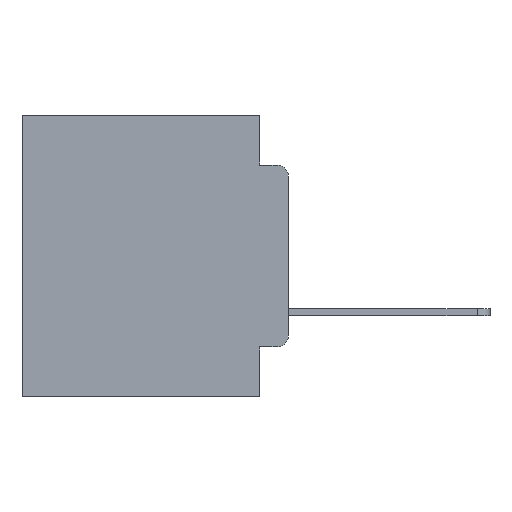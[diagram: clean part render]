
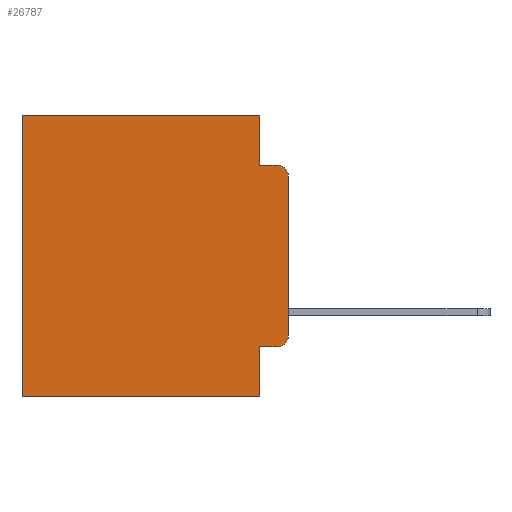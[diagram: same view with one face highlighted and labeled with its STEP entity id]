
A CAD part, left-side view. The second image highlights one B-rep face of the part: STEP entity #26787.
In plain terms, the highlighted planar face has unit normal (-1, 0, 0).
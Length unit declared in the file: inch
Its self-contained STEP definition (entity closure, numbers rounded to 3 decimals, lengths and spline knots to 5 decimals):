
#44 = CARTESIAN_POINT ( 'NONE',  ( 0.298, 0., -0.5 ) ) ;
#45 = EDGE_CURVE ( 'NONE', #5081, #11449, #20028, .T. ) ;
#139 = DIRECTION ( 'NONE',  ( 0., 1., 0. ) ) ;
#180 = VERTEX_POINT ( 'NONE', #13014 ) ;
#306 = ORIENTED_EDGE ( 'NONE', *, *, #12831, .F. ) ;
#857 = EDGE_CURVE ( 'NONE', #6445, #17383, #17025, .T. ) ;
#1104 = VECTOR ( 'NONE', #11165, 39.37008 ) ;
#1375 = VERTEX_POINT ( 'NONE', #20201 ) ;
#2165 = VECTOR ( 'NONE', #139, 39.37008 ) ;
#2789 = CARTESIAN_POINT ( 'NONE',  ( 0.298, 0., -0.3915 ) ) ;
#2856 = LINE ( 'NONE', #44, #2165 ) ;
#3295 = EDGE_CURVE ( 'NONE', #11449, #10520, #14204, .T. ) ;
#4187 = CIRCLE ( 'NONE', #17634, 0.02 ) ;
#4429 = AXIS2_PLACEMENT_3D ( 'NONE', #17873, #19975, #7284 ) ;
#5081 = VERTEX_POINT ( 'NONE', #22163 ) ;
#5127 = FACE_OUTER_BOUND ( 'NONE', #22429, .T. ) ;
#5281 = CARTESIAN_POINT ( 'NONE',  ( 0.298, 0.02, -0.4115 ) ) ;
#5890 = DIRECTION ( 'NONE',  ( 0., -1., 0. ) ) ;
#5969 = CARTESIAN_POINT ( 'NONE',  ( 0.298, 0., 0. ) ) ;
#6206 = ORIENTED_EDGE ( 'NONE', *, *, #22382, .F. ) ;
#6445 = VERTEX_POINT ( 'NONE', #11543 ) ;
#6539 = DIRECTION ( 'NONE',  ( 0., 1., 0. ) ) ;
#6581 = ORIENTED_EDGE ( 'NONE', *, *, #3295, .T. ) ;
#6962 = VECTOR ( 'NONE', #25093, 39.37008 ) ;
#7270 = DIRECTION ( 'NONE',  ( 0., 0., -1. ) ) ;
#7284 = DIRECTION ( 'NONE',  ( 0., 0., -1. ) ) ;
#7630 = LINE ( 'NONE', #10221, #6962 ) ;
#8241 = EDGE_CURVE ( 'NONE', #6445, #21262, #14792, .T. ) ;
#8368 = VERTEX_POINT ( 'NONE', #2789 ) ;
#8591 = EDGE_CURVE ( 'NONE', #180, #22905, #16775, .T. ) ;
#8826 = CARTESIAN_POINT ( 'NONE',  ( 0.298, 0.02, -0.0885 ) ) ;
#8924 = DIRECTION ( 'NONE',  ( -1., 0., 0. ) ) ;
#9073 = CARTESIAN_POINT ( 'NONE',  ( 0.298, 0.051, 0. ) ) ;
#9126 = VECTOR ( 'NONE', #17661, 39.37008 ) ;
#10221 = CARTESIAN_POINT ( 'NONE',  ( 0.298, 0., 0. ) ) ;
#10312 = CARTESIAN_POINT ( 'NONE',  ( 0.298, 0.473, -0.5 ) ) ;
#10520 = VERTEX_POINT ( 'NONE', #10312 ) ;
#11049 = VECTOR ( 'NONE', #5890, 39.37008 ) ;
#11165 = DIRECTION ( 'NONE',  ( 0., 0., -1. ) ) ;
#11226 = EDGE_CURVE ( 'NONE', #17383, #10520, #2856, .T. ) ;
#11449 = VERTEX_POINT ( 'NONE', #22228 ) ;
#11543 = CARTESIAN_POINT ( 'NONE',  ( 0.298, 0.051, -0.4115 ) ) ;
#11707 = CIRCLE ( 'NONE', #12276, 0.02 ) ;
#12091 = DIRECTION ( 'NONE',  ( -1., 0., 0. ) ) ;
#12147 = ORIENTED_EDGE ( 'NONE', *, *, #16267, .T. ) ;
#12276 = AXIS2_PLACEMENT_3D ( 'NONE', #24764, #12091, #26854 ) ;
#12831 = EDGE_CURVE ( 'NONE', #1375, #8368, #7630, .T. ) ;
#12913 = ORIENTED_EDGE ( 'NONE', *, *, #22917, .T. ) ;
#13014 = CARTESIAN_POINT ( 'NONE',  ( 0.298, 0.051, -0.0885 ) ) ;
#14204 = LINE ( 'NONE', #21202, #25377 ) ;
#14382 = VECTOR ( 'NONE', #6539, 39.37008 ) ;
#14792 = LINE ( 'NONE', #25942, #9126 ) ;
#15747 = PLANE ( 'NONE',  #4429 ) ;
#16267 = EDGE_CURVE ( 'NONE', #1375, #22905, #11707, .T. ) ;
#16775 = LINE ( 'NONE', #22837, #11049 ) ;
#16961 = ORIENTED_EDGE ( 'NONE', *, *, #8241, .T. ) ;
#17025 = LINE ( 'NONE', #19109, #27463 ) ;
#17383 = VERTEX_POINT ( 'NONE', #27240 ) ;
#17634 = AXIS2_PLACEMENT_3D ( 'NONE', #21609, #8924, #23697 ) ;
#17661 = DIRECTION ( 'NONE',  ( 0., -1., 0. ) ) ;
#17873 = CARTESIAN_POINT ( 'NONE',  ( 0.298, 0., 0. ) ) ;
#19109 = CARTESIAN_POINT ( 'NONE',  ( 0.298, 0.051, 0. ) ) ;
#19975 = DIRECTION ( 'NONE',  ( 1., 0., 0. ) ) ;
#20028 = LINE ( 'NONE', #5969, #14382 ) ;
#20201 = CARTESIAN_POINT ( 'NONE',  ( 0.298, 0., -0.1085 ) ) ;
#20206 = ORIENTED_EDGE ( 'NONE', *, *, #857, .F. ) ;
#20669 = ORIENTED_EDGE ( 'NONE', *, *, #8591, .F. ) ;
#21202 = CARTESIAN_POINT ( 'NONE',  ( 0.298, 0.473, 0. ) ) ;
#21262 = VERTEX_POINT ( 'NONE', #5281 ) ;
#21609 = CARTESIAN_POINT ( 'NONE',  ( 0.298, 0.02, -0.3915 ) ) ;
#21822 = ORIENTED_EDGE ( 'NONE', *, *, #45, .T. ) ;
#22163 = CARTESIAN_POINT ( 'NONE',  ( 0.298, 0.051, 0. ) ) ;
#22228 = CARTESIAN_POINT ( 'NONE',  ( 0.298, 0.473, 0. ) ) ;
#22382 = EDGE_CURVE ( 'NONE', #5081, #180, #22519, .T. ) ;
#22429 = EDGE_LOOP ( 'NONE', ( #306, #12147, #20669, #6206, #21822, #6581, #23802, #20206, #16961, #12913 ) ) ;
#22496 = DIRECTION ( 'NONE',  ( 0., 0., -1. ) ) ;
#22519 = LINE ( 'NONE', #9073, #1104 ) ;
#22837 = CARTESIAN_POINT ( 'NONE',  ( 0.298, 0.051, -0.0885 ) ) ;
#22905 = VERTEX_POINT ( 'NONE', #8826 ) ;
#22917 = EDGE_CURVE ( 'NONE', #21262, #8368, #4187, .T. ) ;
#23697 = DIRECTION ( 'NONE',  ( 0., 0., -1. ) ) ;
#23802 = ORIENTED_EDGE ( 'NONE', *, *, #11226, .F. ) ;
#24764 = CARTESIAN_POINT ( 'NONE',  ( 0.298, 0.02, -0.1085 ) ) ;
#25093 = DIRECTION ( 'NONE',  ( 0., 0., -1. ) ) ;
#25377 = VECTOR ( 'NONE', #7270, 39.37008 ) ;
#25942 = CARTESIAN_POINT ( 'NONE',  ( 0.298, 0.051, -0.4115 ) ) ;
#26787 = ADVANCED_FACE ( 'NONE', ( #5127 ), #15747, .F. ) ;
#26854 = DIRECTION ( 'NONE',  ( 0., 0., -1. ) ) ;
#27240 = CARTESIAN_POINT ( 'NONE',  ( 0.298, 0.051, -0.5 ) ) ;
#27463 = VECTOR ( 'NONE', #22496, 39.37008 ) ;
